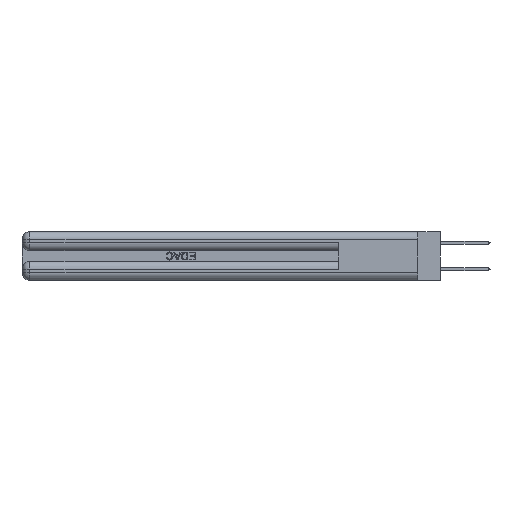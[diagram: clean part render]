
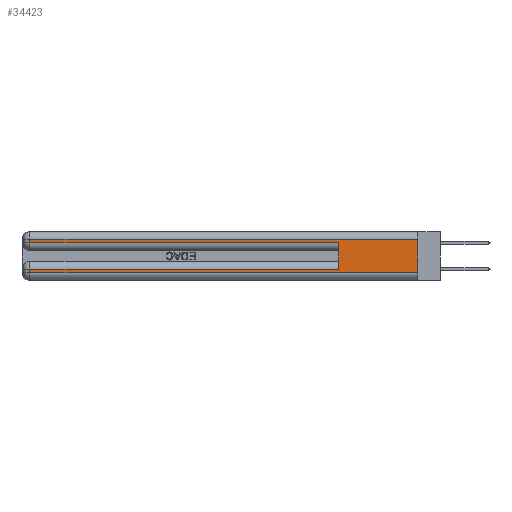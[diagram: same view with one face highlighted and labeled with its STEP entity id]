
A CAD part, left-side view. The second image highlights one B-rep face of the part: STEP entity #34423.
In plain terms, the highlighted planar face has unit normal (-1, 0, 0).
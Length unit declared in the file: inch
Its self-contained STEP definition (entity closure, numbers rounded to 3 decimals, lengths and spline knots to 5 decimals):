
#2837 = CARTESIAN_POINT ( 'NONE',  ( 0., 0., 0.06 ) ) ;
#3141 = LINE ( 'NONE', #2837, #14622 ) ;
#3159 = CARTESIAN_POINT ( 'NONE',  ( 0., 2.94, 0.085 ) ) ;
#3720 = CARTESIAN_POINT ( 'NONE',  ( 0., 0., 0.31 ) ) ;
#4062 = ORIENTED_EDGE ( 'NONE', *, *, #28632, .T. ) ;
#4105 = EDGE_CURVE ( 'NONE', #25225, #21957, #6584, .T. ) ;
#5777 = ORIENTED_EDGE ( 'NONE', *, *, #29597, .T. ) ;
#6584 = LINE ( 'NONE', #16418, #30214 ) ;
#7048 = LINE ( 'NONE', #23193, #19159 ) ;
#7098 = DIRECTION ( 'NONE',  ( 0., 0., -1. ) ) ;
#8168 = VECTOR ( 'NONE', #44421, 39.37008 ) ;
#8195 = CARTESIAN_POINT ( 'NONE',  ( 0., 0., 0.06 ) ) ;
#10445 = ORIENTED_EDGE ( 'NONE', *, *, #26293, .T. ) ;
#10481 = PLANE ( 'NONE',  #28263 ) ;
#10544 = CARTESIAN_POINT ( 'NONE',  ( 0., 2.94, 0.285 ) ) ;
#10642 = CARTESIAN_POINT ( 'NONE',  ( 0., 0., 0.37 ) ) ;
#11660 = ORIENTED_EDGE ( 'NONE', *, *, #4105, .T. ) ;
#12594 = ORIENTED_EDGE ( 'NONE', *, *, #12704, .F. ) ;
#12704 = EDGE_CURVE ( 'NONE', #34285, #27395, #7048, .T. ) ;
#14622 = VECTOR ( 'NONE', #34892, 39.37008 ) ;
#14709 = EDGE_LOOP ( 'NONE', ( #30498, #11660, #5777, #35796, #12594, #34130, #4062, #10445 ) ) ;
#15622 = LINE ( 'NONE', #10642, #43639 ) ;
#16418 = CARTESIAN_POINT ( 'NONE',  ( 0., 0., 0.31 ) ) ;
#16465 = CARTESIAN_POINT ( 'NONE',  ( 0., 0., 0.085 ) ) ;
#17057 = CARTESIAN_POINT ( 'NONE',  ( 0., 0.6, 0.285 ) ) ;
#17148 = DIRECTION ( 'NONE',  ( 1., 0., 0. ) ) ;
#17963 = FACE_OUTER_BOUND ( 'NONE', #14709, .T. ) ;
#19159 = VECTOR ( 'NONE', #37627, 39.37008 ) ;
#19787 = CARTESIAN_POINT ( 'NONE',  ( 0., 0.6, 0.085 ) ) ;
#20269 = CARTESIAN_POINT ( 'NONE',  ( 0., 2.94, 0.06 ) ) ;
#21000 = LINE ( 'NONE', #33526, #30911 ) ;
#21957 = VERTEX_POINT ( 'NONE', #34506 ) ;
#23193 = CARTESIAN_POINT ( 'NONE',  ( 0., 0.6, 0.145 ) ) ;
#23805 = EDGE_CURVE ( 'NONE', #25225, #40407, #15622, .T. ) ;
#24659 = EDGE_CURVE ( 'NONE', #25993, #27395, #21000, .T. ) ;
#25225 = VERTEX_POINT ( 'NONE', #3720 ) ;
#25993 = VERTEX_POINT ( 'NONE', #10544 ) ;
#26293 = EDGE_CURVE ( 'NONE', #31069, #40407, #3141, .T. ) ;
#27395 = VERTEX_POINT ( 'NONE', #17057 ) ;
#28263 = AXIS2_PLACEMENT_3D ( 'NONE', #38200, #17148, #7098 ) ;
#28632 = EDGE_CURVE ( 'NONE', #32798, #31069, #39112, .T. ) ;
#29597 = EDGE_CURVE ( 'NONE', #21957, #25993, #30257, .T. ) ;
#29806 = VECTOR ( 'NONE', #30732, 39.37008 ) ;
#30214 = VECTOR ( 'NONE', #30520, 39.37008 ) ;
#30257 = LINE ( 'NONE', #42870, #32955 ) ;
#30498 = ORIENTED_EDGE ( 'NONE', *, *, #23805, .F. ) ;
#30520 = DIRECTION ( 'NONE',  ( 0., 1., 0. ) ) ;
#30732 = DIRECTION ( 'NONE',  ( 0., 0., -1. ) ) ;
#30911 = VECTOR ( 'NONE', #39955, 39.37008 ) ;
#31069 = VERTEX_POINT ( 'NONE', #20269 ) ;
#31313 = LINE ( 'NONE', #16465, #8168 ) ;
#32101 = DIRECTION ( 'NONE',  ( 0., 0., -1. ) ) ;
#32798 = VERTEX_POINT ( 'NONE', #3159 ) ;
#32955 = VECTOR ( 'NONE', #32101, 39.37008 ) ;
#33526 = CARTESIAN_POINT ( 'NONE',  ( 0., 0., 0.285 ) ) ;
#34130 = ORIENTED_EDGE ( 'NONE', *, *, #39964, .T. ) ;
#34285 = VERTEX_POINT ( 'NONE', #19787 ) ;
#34423 = ADVANCED_FACE ( 'NONE', ( #17963 ), #10481, .F. ) ;
#34506 = CARTESIAN_POINT ( 'NONE',  ( 0., 2.94, 0.31 ) ) ;
#34892 = DIRECTION ( 'NONE',  ( 0., -1., 0. ) ) ;
#35796 = ORIENTED_EDGE ( 'NONE', *, *, #24659, .T. ) ;
#37627 = DIRECTION ( 'NONE',  ( 0., 0., 1. ) ) ;
#38200 = CARTESIAN_POINT ( 'NONE',  ( 0., 0., 0.37 ) ) ;
#38231 = DIRECTION ( 'NONE',  ( 0., 0., -1. ) ) ;
#39112 = LINE ( 'NONE', #44743, #29806 ) ;
#39955 = DIRECTION ( 'NONE',  ( 0., -1., 0. ) ) ;
#39964 = EDGE_CURVE ( 'NONE', #34285, #32798, #31313, .T. ) ;
#40407 = VERTEX_POINT ( 'NONE', #8195 ) ;
#42870 = CARTESIAN_POINT ( 'NONE',  ( 0., 2.94, 0.37 ) ) ;
#43639 = VECTOR ( 'NONE', #38231, 39.37008 ) ;
#44421 = DIRECTION ( 'NONE',  ( 0., 1., 0. ) ) ;
#44743 = CARTESIAN_POINT ( 'NONE',  ( 0., 2.94, 0.37 ) ) ;
